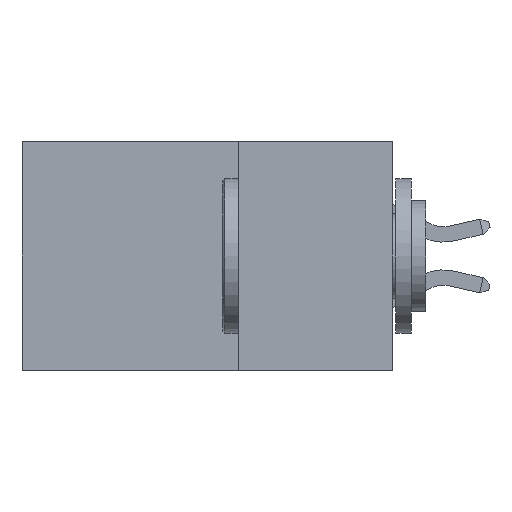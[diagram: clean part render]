
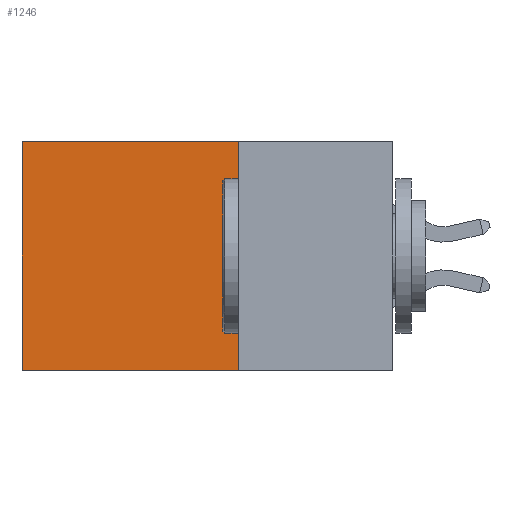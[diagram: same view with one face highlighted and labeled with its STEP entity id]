
A CAD part, left-side view. The second image highlights one B-rep face of the part: STEP entity #1246.
In plain terms, the highlighted planar face has unit normal (-1, 0, 0).
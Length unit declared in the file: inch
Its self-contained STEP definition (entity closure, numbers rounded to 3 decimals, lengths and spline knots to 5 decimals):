
#61 = FACE_OUTER_BOUND ( 'NONE', #1824, .T. ) ;
#85 = VECTOR ( 'NONE', #9674, 39.37008 ) ;
#443 = CARTESIAN_POINT ( 'NONE',  ( 0.2875, 0.25, -0.37 ) ) ;
#1164 = EDGE_CURVE ( 'NONE', #2709, #5525, #4973, .T. ) ;
#1246 = ADVANCED_FACE ( 'NONE', ( #61 ), #9255, .F. ) ;
#1818 = CARTESIAN_POINT ( 'NONE',  ( 0.2875, 0.6, 0. ) ) ;
#1824 = EDGE_LOOP ( 'NONE', ( #6145, #6263, #6618, #6736 ) ) ;
#2260 = CARTESIAN_POINT ( 'NONE',  ( 0.2875, 0.25, 0. ) ) ;
#2496 = DIRECTION ( 'NONE',  ( 0., 0., -1. ) ) ;
#2514 = VERTEX_POINT ( 'NONE', #1818 ) ;
#2565 = CARTESIAN_POINT ( 'NONE',  ( 0.2875, 0.6, 0. ) ) ;
#2709 = VERTEX_POINT ( 'NONE', #5362 ) ;
#3555 = CARTESIAN_POINT ( 'NONE',  ( 0.2875, 0.25, 0. ) ) ;
#3578 = CARTESIAN_POINT ( 'NONE',  ( 0.2875, 0.25, 0. ) ) ;
#3816 = DIRECTION ( 'NONE',  ( 0., 0., -1. ) ) ;
#3901 = VECTOR ( 'NONE', #5864, 39.37008 ) ;
#4148 = LINE ( 'NONE', #3578, #3901 ) ;
#4781 = AXIS2_PLACEMENT_3D ( 'NONE', #2260, #8205, #3816 ) ;
#4827 = CARTESIAN_POINT ( 'NONE',  ( 0.2875, 0.6, -0.37 ) ) ;
#4973 = LINE ( 'NONE', #3555, #8882 ) ;
#5362 = CARTESIAN_POINT ( 'NONE',  ( 0.2875, 0.25, 0. ) ) ;
#5525 = VERTEX_POINT ( 'NONE', #5625 ) ;
#5625 = CARTESIAN_POINT ( 'NONE',  ( 0.2875, 0.25, -0.37 ) ) ;
#5864 = DIRECTION ( 'NONE',  ( 0., 1., 0. ) ) ;
#6109 = EDGE_CURVE ( 'NONE', #2514, #8343, #8810, .T. ) ;
#6145 = ORIENTED_EDGE ( 'NONE', *, *, #6109, .T. ) ;
#6263 = ORIENTED_EDGE ( 'NONE', *, *, #6865, .F. ) ;
#6618 = ORIENTED_EDGE ( 'NONE', *, *, #1164, .F. ) ;
#6736 = ORIENTED_EDGE ( 'NONE', *, *, #9020, .T. ) ;
#6865 = EDGE_CURVE ( 'NONE', #5525, #8343, #8261, .T. ) ;
#7913 = DIRECTION ( 'NONE',  ( 0., 0., -1. ) ) ;
#8205 = DIRECTION ( 'NONE',  ( 1., 0., 0. ) ) ;
#8261 = LINE ( 'NONE', #443, #85 ) ;
#8343 = VERTEX_POINT ( 'NONE', #4827 ) ;
#8600 = VECTOR ( 'NONE', #2496, 39.37008 ) ;
#8810 = LINE ( 'NONE', #2565, #8600 ) ;
#8882 = VECTOR ( 'NONE', #7913, 39.37008 ) ;
#9020 = EDGE_CURVE ( 'NONE', #2709, #2514, #4148, .T. ) ;
#9255 = PLANE ( 'NONE',  #4781 ) ;
#9674 = DIRECTION ( 'NONE',  ( 0., 1., 0. ) ) ;
